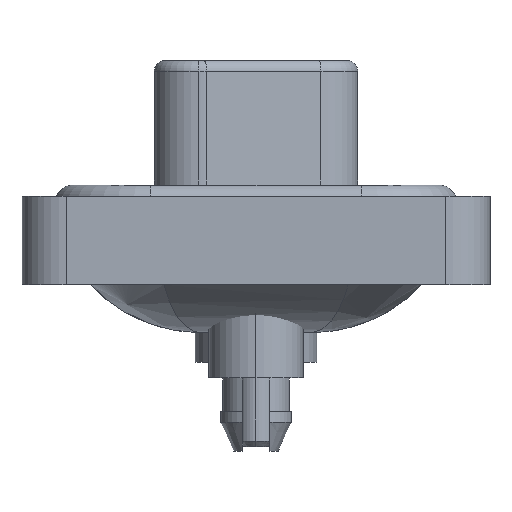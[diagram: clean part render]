
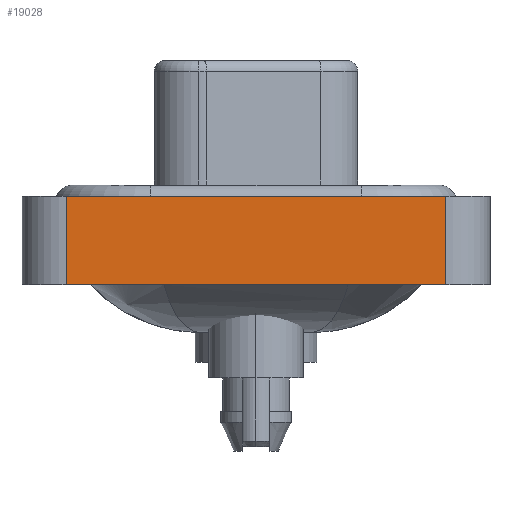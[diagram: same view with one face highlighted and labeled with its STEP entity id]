
A CAD part, left-side view. The second image highlights one B-rep face of the part: STEP entity #19028.
In plain terms, the highlighted planar face has unit normal (-1, 0, 0).
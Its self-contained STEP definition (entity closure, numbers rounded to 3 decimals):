
#59 = EDGE_LOOP ( 'NONE', ( #6624, #8140, #7583, #4847 ) ) ;
#331 = DIRECTION ( 'NONE',  ( -1., 0., 0. ) ) ;
#574 = CARTESIAN_POINT ( 'NONE',  ( -7.3, 8.55, -3.6 ) ) ;
#920 = AXIS2_PLACEMENT_3D ( 'NONE', #4913, #331, #5025 ) ;
#1668 = CARTESIAN_POINT ( 'NONE',  ( -7.3, -8.55, 0.4 ) ) ;
#1856 = EDGE_CURVE ( 'NONE', #9569, #21423, #9615, .T. ) ;
#2207 = CARTESIAN_POINT ( 'NONE',  ( -7.3, 8.55, 0.4 ) ) ;
#2438 = LINE ( 'NONE', #9074, #20559 ) ;
#4208 = CARTESIAN_POINT ( 'NONE',  ( -7.3, -8.55, -3.6 ) ) ;
#4746 = CARTESIAN_POINT ( 'NONE',  ( -7.3, -8.55, -3.6 ) ) ;
#4847 = ORIENTED_EDGE ( 'NONE', *, *, #10761, .T. ) ;
#4913 = CARTESIAN_POINT ( 'NONE',  ( -7.3, -8.55, -3.6 ) ) ;
#5025 = DIRECTION ( 'NONE',  ( 0., 0., 1. ) ) ;
#6124 = CARTESIAN_POINT ( 'NONE',  ( -7.3, -8.55, 0.4 ) ) ;
#6624 = ORIENTED_EDGE ( 'NONE', *, *, #7766, .T. ) ;
#7583 = ORIENTED_EDGE ( 'NONE', *, *, #12153, .F. ) ;
#7640 = VERTEX_POINT ( 'NONE', #11920 ) ;
#7694 = LINE ( 'NONE', #4746, #11910 ) ;
#7766 = EDGE_CURVE ( 'NONE', #10553, #21423, #2438, .T. ) ;
#8140 = ORIENTED_EDGE ( 'NONE', *, *, #1856, .F. ) ;
#8522 = VECTOR ( 'NONE', #12772, 1000. ) ;
#8763 = VECTOR ( 'NONE', #20679, 1000. ) ;
#9074 = CARTESIAN_POINT ( 'NONE',  ( -7.3, -8.55, -3.6 ) ) ;
#9569 = VERTEX_POINT ( 'NONE', #2207 ) ;
#9615 = LINE ( 'NONE', #6124, #8522 ) ;
#10553 = VERTEX_POINT ( 'NONE', #4208 ) ;
#10761 = EDGE_CURVE ( 'NONE', #7640, #10553, #7694, .T. ) ;
#11910 = VECTOR ( 'NONE', #21248, 1000. ) ;
#11920 = CARTESIAN_POINT ( 'NONE',  ( -7.3, 8.55, -3.6 ) ) ;
#12153 = EDGE_CURVE ( 'NONE', #7640, #9569, #17322, .T. ) ;
#12772 = DIRECTION ( 'NONE',  ( 0., -1., 0. ) ) ;
#15708 = DIRECTION ( 'NONE',  ( 0., 0., 1. ) ) ;
#16334 = FACE_OUTER_BOUND ( 'NONE', #59, .T. ) ;
#17322 = LINE ( 'NONE', #574, #8763 ) ;
#19028 = ADVANCED_FACE ( 'NONE', ( #16334 ), #21425, .T. ) ;
#20559 = VECTOR ( 'NONE', #15708, 1000. ) ;
#20679 = DIRECTION ( 'NONE',  ( 0., 0., 1. ) ) ;
#21248 = DIRECTION ( 'NONE',  ( 0., -1., 0. ) ) ;
#21423 = VERTEX_POINT ( 'NONE', #1668 ) ;
#21425 = PLANE ( 'NONE',  #920 ) ;
